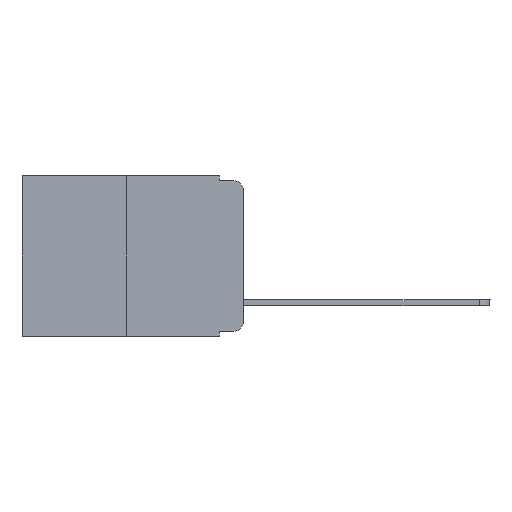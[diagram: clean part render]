
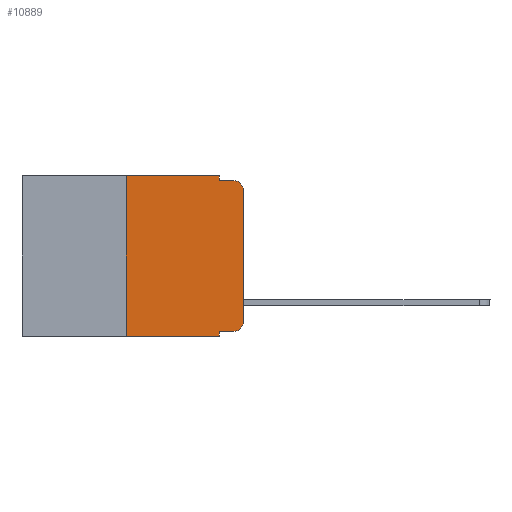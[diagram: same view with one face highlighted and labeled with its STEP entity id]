
A CAD part, left-side view. The second image highlights one B-rep face of the part: STEP entity #10889.
In plain terms, the highlighted planar face has unit normal (-1, 0, 0).
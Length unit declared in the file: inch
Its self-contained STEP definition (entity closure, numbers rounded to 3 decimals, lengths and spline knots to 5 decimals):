
#240 = DIRECTION ( 'NONE',  ( 0., 0., -1. ) ) ;
#259 = CIRCLE ( 'NONE', #19418, 0.02 ) ;
#276 = CARTESIAN_POINT ( 'NONE',  ( 0., 0., 0. ) ) ;
#316 = CARTESIAN_POINT ( 'NONE',  ( 0., 0.02, -0.03 ) ) ;
#752 = LINE ( 'NONE', #6963, #7765 ) ;
#973 = CARTESIAN_POINT ( 'NONE',  ( 0., 0.25, 0. ) ) ;
#1017 = VECTOR ( 'NONE', #5456, 39.37008 ) ;
#1082 = VERTEX_POINT ( 'NONE', #10263 ) ;
#1819 = DIRECTION ( 'NONE',  ( 0., -1., 0. ) ) ;
#2004 = CARTESIAN_POINT ( 'NONE',  ( 0., 0.25, 0. ) ) ;
#2701 = ORIENTED_EDGE ( 'NONE', *, *, #2813, .T. ) ;
#2813 = EDGE_CURVE ( 'NONE', #9075, #17462, #259, .T. ) ;
#2945 = EDGE_CURVE ( 'NONE', #17462, #18077, #22129, .T. ) ;
#2977 = EDGE_LOOP ( 'NONE', ( #18390, #11493, #19293, #6644, #13696, #20001, #3768, #11421, #10942, #2701 ) ) ;
#3635 = EDGE_CURVE ( 'NONE', #8225, #18481, #5845, .T. ) ;
#3705 = VECTOR ( 'NONE', #22877, 39.37008 ) ;
#3768 = ORIENTED_EDGE ( 'NONE', *, *, #16742, .T. ) ;
#3913 = CARTESIAN_POINT ( 'NONE',  ( 0., 0.051, 0. ) ) ;
#3957 = VECTOR ( 'NONE', #7382, 39.37008 ) ;
#4477 = EDGE_CURVE ( 'NONE', #10396, #8225, #752, .T. ) ;
#4499 = VECTOR ( 'NONE', #5131, 39.37008 ) ;
#4933 = VERTEX_POINT ( 'NONE', #20818 ) ;
#4955 = CARTESIAN_POINT ( 'NONE',  ( 0., 0.051, -0.333 ) ) ;
#4984 = CARTESIAN_POINT ( 'NONE',  ( 0., 0.473, 0. ) ) ;
#5131 = DIRECTION ( 'NONE',  ( 0., -1., 0. ) ) ;
#5154 = DIRECTION ( 'NONE',  ( 0., -1., 0. ) ) ;
#5158 = DIRECTION ( 'NONE',  ( 0., 0., -1. ) ) ;
#5456 = DIRECTION ( 'NONE',  ( 0., 0., 1. ) ) ;
#5778 = CIRCLE ( 'NONE', #6299, 0.02 ) ;
#5845 = LINE ( 'NONE', #15859, #19588 ) ;
#6299 = AXIS2_PLACEMENT_3D ( 'NONE', #316, #12818, #240 ) ;
#6482 = AXIS2_PLACEMENT_3D ( 'NONE', #21085, #12973, #16360 ) ;
#6644 = ORIENTED_EDGE ( 'NONE', *, *, #4477, .F. ) ;
#6898 = DIRECTION ( 'NONE',  ( -1., 0., 0. ) ) ;
#6963 = CARTESIAN_POINT ( 'NONE',  ( 0., 0.051, 0. ) ) ;
#7203 = CARTESIAN_POINT ( 'NONE',  ( 0., 0.02, -0.313 ) ) ;
#7217 = CARTESIAN_POINT ( 'NONE',  ( 0., 0.473, -0.343 ) ) ;
#7382 = DIRECTION ( 'NONE',  ( 0., 0., -1. ) ) ;
#7765 = VECTOR ( 'NONE', #15775, 39.37008 ) ;
#8225 = VERTEX_POINT ( 'NONE', #16143 ) ;
#8656 = PLANE ( 'NONE',  #6482 ) ;
#9075 = VERTEX_POINT ( 'NONE', #16379 ) ;
#9121 = CARTESIAN_POINT ( 'NONE',  ( 0., 0.051, -0.343 ) ) ;
#9300 = EDGE_CURVE ( 'NONE', #1082, #10742, #20214, .T. ) ;
#9830 = FACE_OUTER_BOUND ( 'NONE', #2977, .T. ) ;
#10263 = CARTESIAN_POINT ( 'NONE',  ( 0., 0.051, -0.333 ) ) ;
#10396 = VERTEX_POINT ( 'NONE', #20013 ) ;
#10742 = VERTEX_POINT ( 'NONE', #9121 ) ;
#10889 = ADVANCED_FACE ( 'NONE', ( #9830 ), #8656, .F. ) ;
#10942 = ORIENTED_EDGE ( 'NONE', *, *, #20560, .T. ) ;
#11177 = CARTESIAN_POINT ( 'NONE',  ( 0., 0., -0.03 ) ) ;
#11421 = ORIENTED_EDGE ( 'NONE', *, *, #9300, .F. ) ;
#11493 = ORIENTED_EDGE ( 'NONE', *, *, #16653, .T. ) ;
#12675 = VERTEX_POINT ( 'NONE', #973 ) ;
#12818 = DIRECTION ( 'NONE',  ( -1., 0., 0. ) ) ;
#12937 = LINE ( 'NONE', #4955, #3705 ) ;
#12973 = DIRECTION ( 'NONE',  ( 1., 0., 0. ) ) ;
#13530 = EDGE_CURVE ( 'NONE', #12675, #10396, #13974, .T. ) ;
#13696 = ORIENTED_EDGE ( 'NONE', *, *, #13530, .F. ) ;
#13974 = LINE ( 'NONE', #4984, #4499 ) ;
#15775 = DIRECTION ( 'NONE',  ( 0., 0., -1. ) ) ;
#15859 = CARTESIAN_POINT ( 'NONE',  ( 0., 0.051, -0.01 ) ) ;
#16143 = CARTESIAN_POINT ( 'NONE',  ( 0., 0.051, -0.01 ) ) ;
#16360 = DIRECTION ( 'NONE',  ( 0., 0., -1. ) ) ;
#16379 = CARTESIAN_POINT ( 'NONE',  ( 0., 0.02, -0.333 ) ) ;
#16653 = EDGE_CURVE ( 'NONE', #18077, #18481, #5778, .T. ) ;
#16714 = CARTESIAN_POINT ( 'NONE',  ( 0., 0., -0.313 ) ) ;
#16742 = EDGE_CURVE ( 'NONE', #4933, #10742, #20911, .T. ) ;
#17391 = VECTOR ( 'NONE', #21731, 39.37008 ) ;
#17462 = VERTEX_POINT ( 'NONE', #16714 ) ;
#18077 = VERTEX_POINT ( 'NONE', #11177 ) ;
#18390 = ORIENTED_EDGE ( 'NONE', *, *, #2945, .T. ) ;
#18481 = VERTEX_POINT ( 'NONE', #21289 ) ;
#19076 = EDGE_CURVE ( 'NONE', #4933, #12675, #20041, .T. ) ;
#19293 = ORIENTED_EDGE ( 'NONE', *, *, #3635, .F. ) ;
#19418 = AXIS2_PLACEMENT_3D ( 'NONE', #7203, #6898, #5158 ) ;
#19588 = VECTOR ( 'NONE', #5154, 39.37008 ) ;
#20001 = ORIENTED_EDGE ( 'NONE', *, *, #19076, .F. ) ;
#20013 = CARTESIAN_POINT ( 'NONE',  ( 0., 0.051, 0. ) ) ;
#20041 = LINE ( 'NONE', #2004, #1017 ) ;
#20214 = LINE ( 'NONE', #3913, #3957 ) ;
#20560 = EDGE_CURVE ( 'NONE', #1082, #9075, #12937, .T. ) ;
#20818 = CARTESIAN_POINT ( 'NONE',  ( 0., 0.25, -0.343 ) ) ;
#20911 = LINE ( 'NONE', #7217, #21467 ) ;
#21085 = CARTESIAN_POINT ( 'NONE',  ( 0., 0.473, 0. ) ) ;
#21289 = CARTESIAN_POINT ( 'NONE',  ( 0., 0.02, -0.01 ) ) ;
#21467 = VECTOR ( 'NONE', #1819, 39.37008 ) ;
#21731 = DIRECTION ( 'NONE',  ( 0., 0., 1. ) ) ;
#22129 = LINE ( 'NONE', #276, #17391 ) ;
#22877 = DIRECTION ( 'NONE',  ( 0., -1., 0. ) ) ;
